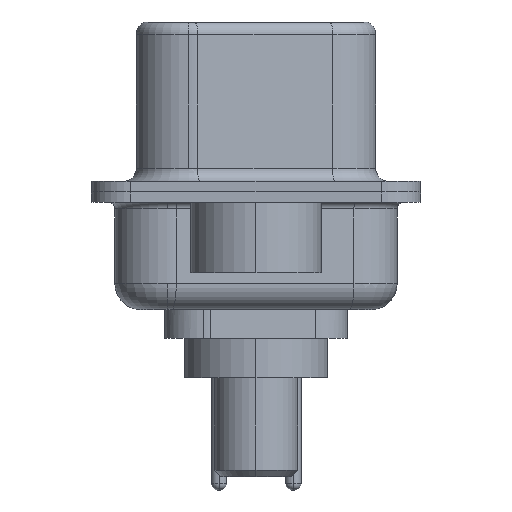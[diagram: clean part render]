
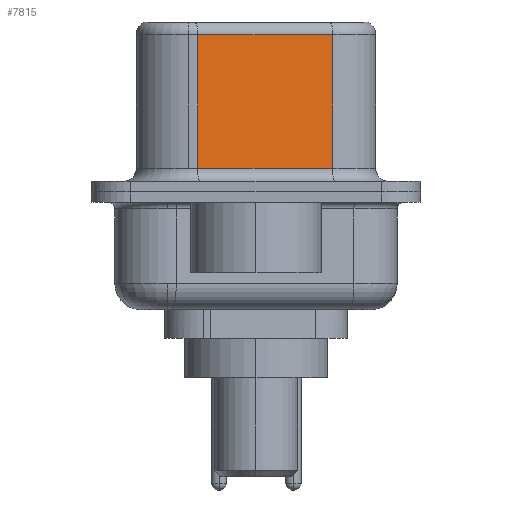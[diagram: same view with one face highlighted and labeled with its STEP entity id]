
A CAD part, left-side view. The second image highlights one B-rep face of the part: STEP entity #7815.
In plain terms, the highlighted planar face has unit normal (-0.985, -0.174, 0).
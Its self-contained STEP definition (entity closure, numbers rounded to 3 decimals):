
#325 = CARTESIAN_POINT ( 'NONE',  ( 3.675, 2.233, 6.02 ) ) ;
#559 = CARTESIAN_POINT ( 'NONE',  ( 3.675, 2.233, 0.9 ) ) ;
#1445 = ORIENTED_EDGE ( 'NONE', *, *, #5324, .T. ) ;
#1541 = LINE ( 'NONE', #5605, #13755 ) ;
#1580 = VECTOR ( 'NONE', #11756, 1000. ) ;
#2148 = ORIENTED_EDGE ( 'NONE', *, *, #10735, .F. ) ;
#2423 = EDGE_CURVE ( 'NONE', #9796, #17365, #19083, .T. ) ;
#2563 = CARTESIAN_POINT ( 'NONE',  ( 3.675, 2.233, 6.52 ) ) ;
#3722 = DIRECTION ( 'NONE',  ( -0.174, 0.985, 0. ) ) ;
#5324 = EDGE_CURVE ( 'NONE', #13277, #12593, #1541, .T. ) ;
#5605 = CARTESIAN_POINT ( 'NONE',  ( 4.585, -2.927, 6.02 ) ) ;
#6265 = VECTOR ( 'NONE', #6580, 1000. ) ;
#6580 = DIRECTION ( 'NONE',  ( 0.174, -0.985, 0. ) ) ;
#6759 = CARTESIAN_POINT ( 'NONE',  ( 4.585, -2.927, 6.02 ) ) ;
#7315 = CARTESIAN_POINT ( 'NONE',  ( 4.585, -2.927, 0.9 ) ) ;
#7815 = ADVANCED_FACE ( 'NONE', ( #11761 ), #19080, .F. ) ;
#9796 = VERTEX_POINT ( 'NONE', #559 ) ;
#10162 = DIRECTION ( 'NONE',  ( -0.174, 0.985, 0. ) ) ;
#10735 = EDGE_CURVE ( 'NONE', #13277, #17365, #19368, .T. ) ;
#11756 = DIRECTION ( 'NONE',  ( 0., 0., -1. ) ) ;
#11761 = FACE_OUTER_BOUND ( 'NONE', #15297, .T. ) ;
#12593 = VERTEX_POINT ( 'NONE', #325 ) ;
#12938 = DIRECTION ( 'NONE',  ( 0.985, 0.174, 0. ) ) ;
#13277 = VERTEX_POINT ( 'NONE', #6759 ) ;
#13326 = LINE ( 'NONE', #2563, #1580 ) ;
#13755 = VECTOR ( 'NONE', #10162, 1000. ) ;
#14100 = EDGE_CURVE ( 'NONE', #12593, #9796, #13326, .T. ) ;
#15085 = CARTESIAN_POINT ( 'NONE',  ( 4.585, -2.927, 6.52 ) ) ;
#15239 = VECTOR ( 'NONE', #16641, 1000. ) ;
#15297 = EDGE_LOOP ( 'NONE', ( #2148, #1445, #17511, #18807 ) ) ;
#15691 = CARTESIAN_POINT ( 'NONE',  ( 4.585, -2.927, 0.9 ) ) ;
#16435 = AXIS2_PLACEMENT_3D ( 'NONE', #19015, #12938, #3722 ) ;
#16641 = DIRECTION ( 'NONE',  ( 0., 0., -1. ) ) ;
#17365 = VERTEX_POINT ( 'NONE', #15691 ) ;
#17511 = ORIENTED_EDGE ( 'NONE', *, *, #14100, .T. ) ;
#18807 = ORIENTED_EDGE ( 'NONE', *, *, #2423, .T. ) ;
#19015 = CARTESIAN_POINT ( 'NONE',  ( 4.585, -2.927, 6.52 ) ) ;
#19080 = PLANE ( 'NONE',  #16435 ) ;
#19083 = LINE ( 'NONE', #7315, #6265 ) ;
#19368 = LINE ( 'NONE', #15085, #15239 ) ;
